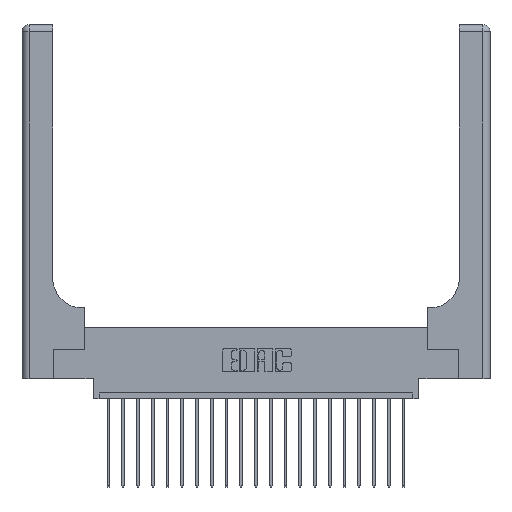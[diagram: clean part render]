
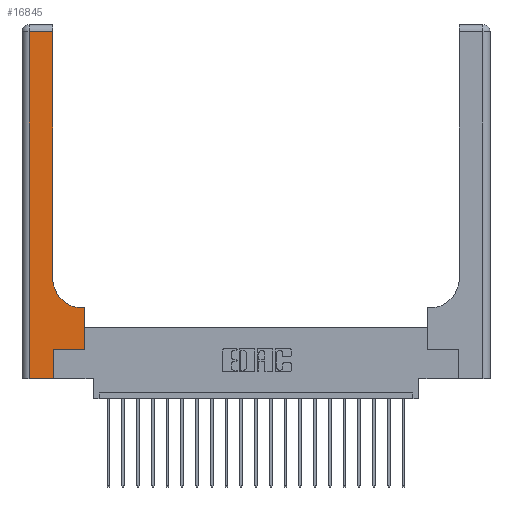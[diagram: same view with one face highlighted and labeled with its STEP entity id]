
A CAD part, top view. The second image highlights one B-rep face of the part: STEP entity #16845.
In plain terms, the highlighted planar face has unit normal (0, 0, 1).
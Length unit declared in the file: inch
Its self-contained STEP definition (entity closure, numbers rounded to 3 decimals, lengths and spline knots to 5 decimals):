
#739 = EDGE_CURVE ( 'NONE', #13040, #14358, #1081, .T. ) ;
#786 = DIRECTION ( 'NONE',  ( 0., 0., -1. ) ) ;
#906 = CARTESIAN_POINT ( 'NONE',  ( 0.51, 0.85, 0.37 ) ) ;
#1070 = LINE ( 'NONE', #6424, #10097 ) ;
#1081 = LINE ( 'NONE', #9611, #21151 ) ;
#1179 = EDGE_LOOP ( 'NONE', ( #9217, #15226, #20805, #1493, #13907, #19350, #20999, #17246, #2117 ) ) ;
#1272 = CARTESIAN_POINT ( 'NONE',  ( 0.265, 0.25, 0.37 ) ) ;
#1493 = ORIENTED_EDGE ( 'NONE', *, *, #5969, .T. ) ;
#1660 = CARTESIAN_POINT ( 'NONE',  ( 0.26, 2.94, 0.37 ) ) ;
#1769 = EDGE_CURVE ( 'NONE', #17935, #4722, #17210, .T. ) ;
#2117 = ORIENTED_EDGE ( 'NONE', *, *, #15233, .T. ) ;
#2315 = CARTESIAN_POINT ( 'NONE',  ( 0.528, 0.25, 0.37 ) ) ;
#2859 = AXIS2_PLACEMENT_3D ( 'NONE', #17412, #786, #7147 ) ;
#3487 = CARTESIAN_POINT ( 'NONE',  ( 0.265, 0.25, 0.37 ) ) ;
#3555 = EDGE_CURVE ( 'NONE', #4722, #7628, #11669, .T. ) ;
#3787 = VERTEX_POINT ( 'NONE', #13750 ) ;
#4147 = EDGE_CURVE ( 'NONE', #20018, #9258, #12594, .T. ) ;
#4544 = AXIS2_PLACEMENT_3D ( 'NONE', #906, #9836, #14356 ) ;
#4690 = EDGE_CURVE ( 'NONE', #14358, #20018, #16271, .T. ) ;
#4722 = VERTEX_POINT ( 'NONE', #5218 ) ;
#4775 = CARTESIAN_POINT ( 'NONE',  ( 0.06, 3., 0.37 ) ) ;
#5058 = CARTESIAN_POINT ( 'NONE',  ( 0.528, 0.6, 0.37 ) ) ;
#5218 = CARTESIAN_POINT ( 'NONE',  ( 0.06, 2.94, 0.37 ) ) ;
#5276 = PLANE ( 'NONE',  #2859 ) ;
#5969 = EDGE_CURVE ( 'NONE', #7628, #13040, #1070, .T. ) ;
#5995 = DIRECTION ( 'NONE',  ( 1., 0., 0. ) ) ;
#6424 = CARTESIAN_POINT ( 'NONE',  ( 0., 0., 0.37 ) ) ;
#7147 = DIRECTION ( 'NONE',  ( -1., 0., 0. ) ) ;
#7628 = VERTEX_POINT ( 'NONE', #11971 ) ;
#7935 = VECTOR ( 'NONE', #14819, 39.37008 ) ;
#7945 = DIRECTION ( 'NONE',  ( 1., 0., 0. ) ) ;
#8061 = VERTEX_POINT ( 'NONE', #19126 ) ;
#8670 = EDGE_CURVE ( 'NONE', #3787, #17935, #16453, .T. ) ;
#8759 = VECTOR ( 'NONE', #15062, 39.37008 ) ;
#8785 = VECTOR ( 'NONE', #8978, 39.37008 ) ;
#8978 = DIRECTION ( 'NONE',  ( 0., 1., 0. ) ) ;
#9023 = EDGE_CURVE ( 'NONE', #9258, #8061, #15692, .T. ) ;
#9217 = ORIENTED_EDGE ( 'NONE', *, *, #8670, .T. ) ;
#9258 = VERTEX_POINT ( 'NONE', #5058 ) ;
#9611 = CARTESIAN_POINT ( 'NONE',  ( 0.265, 0., 0.37 ) ) ;
#9836 = DIRECTION ( 'NONE',  ( 0., 0., -1. ) ) ;
#10097 = VECTOR ( 'NONE', #5995, 39.37008 ) ;
#11669 = LINE ( 'NONE', #4775, #8759 ) ;
#11971 = CARTESIAN_POINT ( 'NONE',  ( 0.06, 0., 0.37 ) ) ;
#12594 = LINE ( 'NONE', #2315, #8785 ) ;
#12957 = VECTOR ( 'NONE', #7945, 39.37008 ) ;
#13040 = VERTEX_POINT ( 'NONE', #17497 ) ;
#13750 = CARTESIAN_POINT ( 'NONE',  ( 0.26, 0.85, 0.37 ) ) ;
#13907 = ORIENTED_EDGE ( 'NONE', *, *, #739, .T. ) ;
#13991 = CIRCLE ( 'NONE', #4544, 0.25 ) ;
#14055 = CARTESIAN_POINT ( 'NONE',  ( 0.26, 0.6, 0.37 ) ) ;
#14356 = DIRECTION ( 'NONE',  ( 1., 0., 0. ) ) ;
#14358 = VERTEX_POINT ( 'NONE', #3487 ) ;
#14819 = DIRECTION ( 'NONE',  ( 0., 1., 0. ) ) ;
#15062 = DIRECTION ( 'NONE',  ( 0., -1., 0. ) ) ;
#15226 = ORIENTED_EDGE ( 'NONE', *, *, #1769, .T. ) ;
#15233 = EDGE_CURVE ( 'NONE', #8061, #3787, #13991, .T. ) ;
#15246 = CARTESIAN_POINT ( 'NONE',  ( 0., 2.94, 0.37 ) ) ;
#15692 = LINE ( 'NONE', #14055, #19091 ) ;
#16180 = DIRECTION ( 'NONE',  ( 0., 1., 0. ) ) ;
#16271 = LINE ( 'NONE', #1272, #12957 ) ;
#16453 = LINE ( 'NONE', #19952, #7935 ) ;
#16845 = ADVANCED_FACE ( 'NONE', ( #20702 ), #5276, .F. ) ;
#17099 = DIRECTION ( 'NONE',  ( -1., 0., 0. ) ) ;
#17210 = LINE ( 'NONE', #15246, #21282 ) ;
#17246 = ORIENTED_EDGE ( 'NONE', *, *, #9023, .T. ) ;
#17412 = CARTESIAN_POINT ( 'NONE',  ( 0., 3., 0.37 ) ) ;
#17497 = CARTESIAN_POINT ( 'NONE',  ( 0.265, 0., 0.37 ) ) ;
#17935 = VERTEX_POINT ( 'NONE', #1660 ) ;
#17949 = CARTESIAN_POINT ( 'NONE',  ( 0.528, 0.25, 0.37 ) ) ;
#19091 = VECTOR ( 'NONE', #20724, 39.37008 ) ;
#19126 = CARTESIAN_POINT ( 'NONE',  ( 0.51, 0.6, 0.37 ) ) ;
#19350 = ORIENTED_EDGE ( 'NONE', *, *, #4690, .T. ) ;
#19952 = CARTESIAN_POINT ( 'NONE',  ( 0.26, 3., 0.37 ) ) ;
#20018 = VERTEX_POINT ( 'NONE', #17949 ) ;
#20702 = FACE_OUTER_BOUND ( 'NONE', #1179, .T. ) ;
#20724 = DIRECTION ( 'NONE',  ( -1., 0., 0. ) ) ;
#20805 = ORIENTED_EDGE ( 'NONE', *, *, #3555, .T. ) ;
#20999 = ORIENTED_EDGE ( 'NONE', *, *, #4147, .T. ) ;
#21151 = VECTOR ( 'NONE', #16180, 39.37008 ) ;
#21282 = VECTOR ( 'NONE', #17099, 39.37008 ) ;
